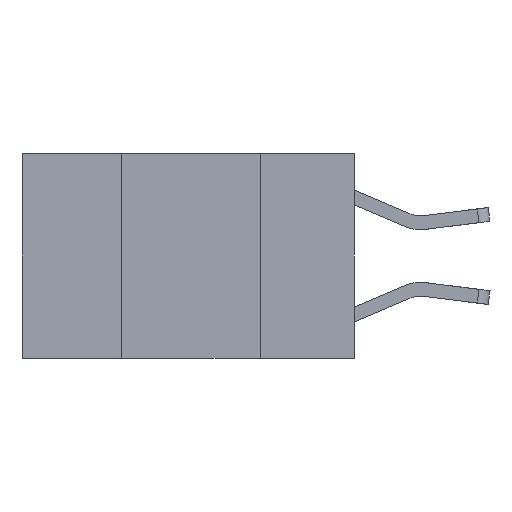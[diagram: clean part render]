
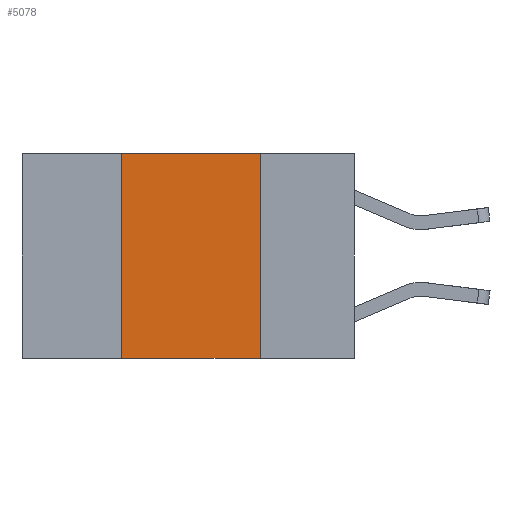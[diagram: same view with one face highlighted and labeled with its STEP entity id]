
A CAD part, left-side view. The second image highlights one B-rep face of the part: STEP entity #5078.
In plain terms, the highlighted planar face has unit normal (-1, 0, 0).
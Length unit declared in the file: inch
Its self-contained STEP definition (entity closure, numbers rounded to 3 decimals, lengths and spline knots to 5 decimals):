
#132 = ORIENTED_EDGE ( 'NONE', *, *, #810, .F. ) ;
#674 = DIRECTION ( 'NONE',  ( 0., 0., -1. ) ) ;
#810 = EDGE_CURVE ( 'NONE', #2326, #2369, #2156, .T. ) ;
#1451 = LINE ( 'NONE', #8513, #8609 ) ;
#1920 = VECTOR ( 'NONE', #6422, 39.37008 ) ;
#2156 = LINE ( 'NONE', #3236, #1920 ) ;
#2210 = PLANE ( 'NONE',  #6109 ) ;
#2218 = CARTESIAN_POINT ( 'NONE',  ( 0., 0.17, -0.37 ) ) ;
#2326 = VERTEX_POINT ( 'NONE', #6042 ) ;
#2369 = VERTEX_POINT ( 'NONE', #3602 ) ;
#2924 = CARTESIAN_POINT ( 'NONE',  ( 0., 0.6, 0. ) ) ;
#2936 = ORIENTED_EDGE ( 'NONE', *, *, #7485, .F. ) ;
#2958 = DIRECTION ( 'NONE',  ( 0., 0., -1. ) ) ;
#3118 = VERTEX_POINT ( 'NONE', #9082 ) ;
#3236 = CARTESIAN_POINT ( 'NONE',  ( 0., 0.6, 0. ) ) ;
#3293 = VECTOR ( 'NONE', #3725, 39.37008 ) ;
#3544 = VERTEX_POINT ( 'NONE', #2218 ) ;
#3602 = CARTESIAN_POINT ( 'NONE',  ( 0., 0.17, 0. ) ) ;
#3725 = DIRECTION ( 'NONE',  ( 0., -1., 0. ) ) ;
#4102 = EDGE_CURVE ( 'NONE', #3118, #3544, #5534, .T. ) ;
#5019 = ORIENTED_EDGE ( 'NONE', *, *, #7749, .F. ) ;
#5078 = ADVANCED_FACE ( 'NONE', ( #8339 ), #2210, .F. ) ;
#5534 = LINE ( 'NONE', #6096, #3293 ) ;
#5919 = ORIENTED_EDGE ( 'NONE', *, *, #4102, .T. ) ;
#6042 = CARTESIAN_POINT ( 'NONE',  ( 0., 0.42, 0. ) ) ;
#6096 = CARTESIAN_POINT ( 'NONE',  ( 0., 0.6, -0.37 ) ) ;
#6109 = AXIS2_PLACEMENT_3D ( 'NONE', #2924, #7072, #2958 ) ;
#6422 = DIRECTION ( 'NONE',  ( 0., -1., 0. ) ) ;
#7065 = EDGE_LOOP ( 'NONE', ( #2936, #132, #5019, #5919 ) ) ;
#7072 = DIRECTION ( 'NONE',  ( 1., 0., 0. ) ) ;
#7147 = DIRECTION ( 'NONE',  ( 0., 0., 1. ) ) ;
#7317 = VECTOR ( 'NONE', #674, 39.37008 ) ;
#7485 = EDGE_CURVE ( 'NONE', #2369, #3544, #8919, .T. ) ;
#7749 = EDGE_CURVE ( 'NONE', #3118, #2326, #1451, .T. ) ;
#8339 = FACE_OUTER_BOUND ( 'NONE', #7065, .T. ) ;
#8404 = CARTESIAN_POINT ( 'NONE',  ( 0., 0.17, 0. ) ) ;
#8513 = CARTESIAN_POINT ( 'NONE',  ( 0., 0.42, 0. ) ) ;
#8609 = VECTOR ( 'NONE', #7147, 39.37008 ) ;
#8919 = LINE ( 'NONE', #8404, #7317 ) ;
#9082 = CARTESIAN_POINT ( 'NONE',  ( 0., 0.42, -0.37 ) ) ;
